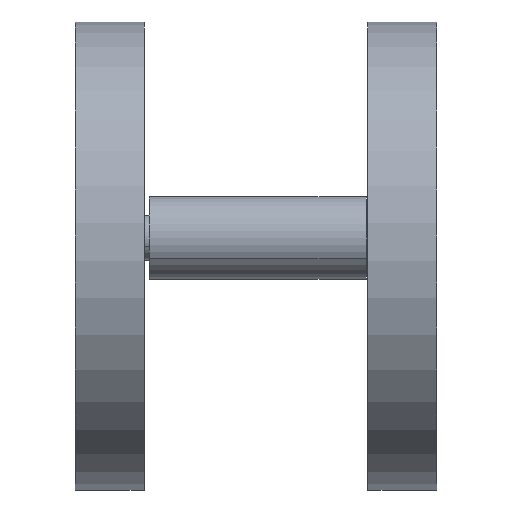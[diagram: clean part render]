
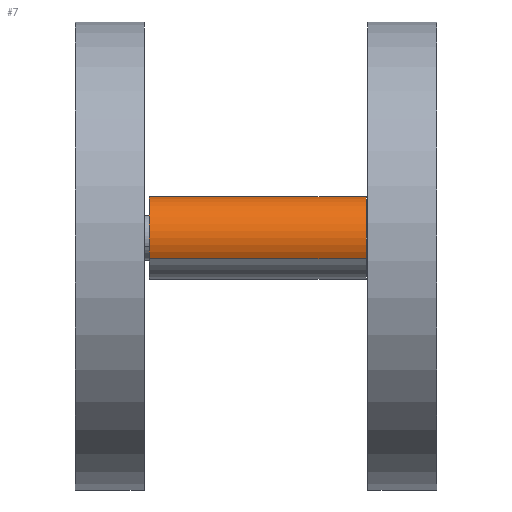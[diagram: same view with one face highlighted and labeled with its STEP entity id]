
A CAD part, top view. The second image highlights one B-rep face of the part: STEP entity #7.
In plain terms, the highlighted cylindrical face has radius 3.048 mm (diameter 6.096 mm), a partial arc.
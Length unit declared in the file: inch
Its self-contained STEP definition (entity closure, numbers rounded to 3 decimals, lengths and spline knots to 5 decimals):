
#2 = ORIENTED_EDGE ( 'NONE', *, *, #903, .T. ) ;
#6 = VECTOR ( 'NONE', #608, 39.37008 ) ;
#7 = ADVANCED_FACE ( 'NONE', ( #503 ), #462, .T. ) ;
#35 = ORIENTED_EDGE ( 'NONE', *, *, #831, .F. ) ;
#53 = EDGE_CURVE ( 'NONE', #897, #80, #357, .T. ) ;
#55 = CARTESIAN_POINT ( 'NONE',  ( 0.12, 0., 0. ) ) ;
#80 = VERTEX_POINT ( 'NONE', #55 ) ;
#131 = VECTOR ( 'NONE', #1188, 39.37008 ) ;
#153 = LINE ( 'NONE', #612, #6 ) ;
#188 = ORIENTED_EDGE ( 'NONE', *, *, #524, .F. ) ;
#261 = DIRECTION ( 'NONE',  ( 0., 0., -1. ) ) ;
#346 = VERTEX_POINT ( 'NONE', #1005 ) ;
#349 = DIRECTION ( 'NONE',  ( -1., 0., 0. ) ) ;
#357 = LINE ( 'NONE', #510, #131 ) ;
#432 = EDGE_LOOP ( 'NONE', ( #188, #1388, #2, #35 ) ) ;
#462 = CYLINDRICAL_SURFACE ( 'NONE', #942, 0.12 ) ;
#498 = CIRCLE ( 'NONE', #1252, 0.12 ) ;
#503 = FACE_OUTER_BOUND ( 'NONE', #432, .T. ) ;
#510 = CARTESIAN_POINT ( 'NONE',  ( 0.12, 0., 0.63 ) ) ;
#524 = EDGE_CURVE ( 'NONE', #897, #346, #498, .T. ) ;
#571 = DIRECTION ( 'NONE',  ( 1., 0., 0. ) ) ;
#572 = DIRECTION ( 'NONE',  ( 0., 0., 1. ) ) ;
#574 = CARTESIAN_POINT ( 'NONE',  ( 0., 0., 0. ) ) ;
#597 = CARTESIAN_POINT ( 'NONE',  ( 0.12, 0., 0.63 ) ) ;
#608 = DIRECTION ( 'NONE',  ( 0., 0., -1. ) ) ;
#612 = CARTESIAN_POINT ( 'NONE',  ( -0.12, 0., 0.63 ) ) ;
#640 = CARTESIAN_POINT ( 'NONE',  ( -0.12, 0., 0. ) ) ;
#741 = VERTEX_POINT ( 'NONE', #640 ) ;
#814 = DIRECTION ( 'NONE',  ( 1., 0., 0. ) ) ;
#816 = DIRECTION ( 'NONE',  ( 0., 0., 1. ) ) ;
#817 = CARTESIAN_POINT ( 'NONE',  ( 0., 0., 0.63 ) ) ;
#831 = EDGE_CURVE ( 'NONE', #346, #741, #153, .T. ) ;
#863 = CIRCLE ( 'NONE', #1099, 0.12 ) ;
#897 = VERTEX_POINT ( 'NONE', #597 ) ;
#903 = EDGE_CURVE ( 'NONE', #80, #741, #863, .T. ) ;
#942 = AXIS2_PLACEMENT_3D ( 'NONE', #1113, #261, #349 ) ;
#1005 = CARTESIAN_POINT ( 'NONE',  ( -0.12, 0., 0.63 ) ) ;
#1099 = AXIS2_PLACEMENT_3D ( 'NONE', #574, #572, #571 ) ;
#1113 = CARTESIAN_POINT ( 'NONE',  ( 0., 0., 0.63 ) ) ;
#1188 = DIRECTION ( 'NONE',  ( 0., 0., -1. ) ) ;
#1252 = AXIS2_PLACEMENT_3D ( 'NONE', #817, #816, #814 ) ;
#1388 = ORIENTED_EDGE ( 'NONE', *, *, #53, .T. ) ;
